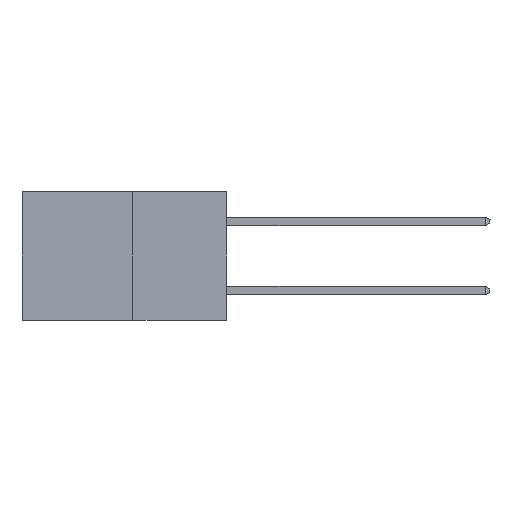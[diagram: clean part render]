
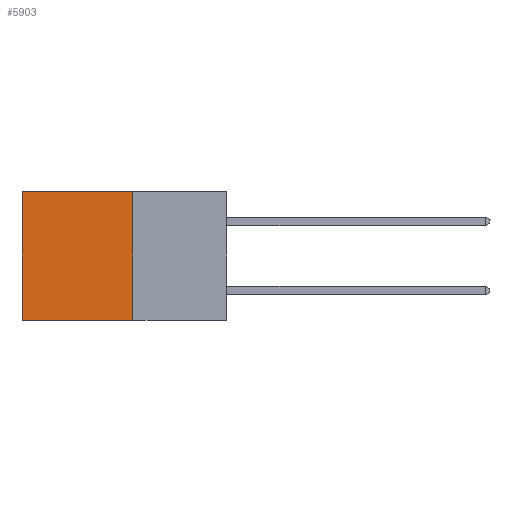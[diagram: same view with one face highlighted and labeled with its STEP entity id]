
A CAD part, left-side view. The second image highlights one B-rep face of the part: STEP entity #5903.
In plain terms, the highlighted planar face has unit normal (-1, 0, 0).
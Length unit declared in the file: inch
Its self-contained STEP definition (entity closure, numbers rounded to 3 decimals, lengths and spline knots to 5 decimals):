
#165 = EDGE_LOOP ( 'NONE', ( #9547, #2135, #2432, #10112 ) ) ;
#430 = DIRECTION ( 'NONE',  ( 0., 1., 0. ) ) ;
#759 = LINE ( 'NONE', #11367, #5685 ) ;
#804 = CARTESIAN_POINT ( 'NONE',  ( 0.277, 0.59, 0. ) ) ;
#1300 = VERTEX_POINT ( 'NONE', #804 ) ;
#1862 = CARTESIAN_POINT ( 'NONE',  ( 0.277, 0.27, -0.37 ) ) ;
#2135 = ORIENTED_EDGE ( 'NONE', *, *, #11477, .F. ) ;
#2406 = EDGE_CURVE ( 'NONE', #11969, #7955, #6826, .T. ) ;
#2407 = CARTESIAN_POINT ( 'NONE',  ( 0.277, 0.27, 0. ) ) ;
#2432 = ORIENTED_EDGE ( 'NONE', *, *, #2406, .F. ) ;
#3671 = DIRECTION ( 'NONE',  ( 0., 0., -1. ) ) ;
#3818 = DIRECTION ( 'NONE',  ( 1., 0., 0. ) ) ;
#5685 = VECTOR ( 'NONE', #10441, 39.37008 ) ;
#5777 = CARTESIAN_POINT ( 'NONE',  ( 0.277, 0.27, -0.37 ) ) ;
#5903 = ADVANCED_FACE ( 'NONE', ( #11142 ), #9595, .F. ) ;
#5915 = AXIS2_PLACEMENT_3D ( 'NONE', #1862, #3818, #10507 ) ;
#6053 = EDGE_CURVE ( 'NONE', #1300, #9940, #9114, .T. ) ;
#6290 = VECTOR ( 'NONE', #430, 39.37008 ) ;
#6358 = CARTESIAN_POINT ( 'NONE',  ( 0.277, 0.27, 0. ) ) ;
#6826 = LINE ( 'NONE', #7202, #11799 ) ;
#6969 = CARTESIAN_POINT ( 'NONE',  ( 0.277, 0.59, -0.37 ) ) ;
#7202 = CARTESIAN_POINT ( 'NONE',  ( 0.277, 0.27, -0.37 ) ) ;
#7955 = VERTEX_POINT ( 'NONE', #5777 ) ;
#8528 = LINE ( 'NONE', #6358, #6290 ) ;
#8804 = VECTOR ( 'NONE', #11646, 39.37008 ) ;
#9114 = LINE ( 'NONE', #6969, #8804 ) ;
#9547 = ORIENTED_EDGE ( 'NONE', *, *, #6053, .T. ) ;
#9595 = PLANE ( 'NONE',  #5915 ) ;
#9940 = VERTEX_POINT ( 'NONE', #10035 ) ;
#10035 = CARTESIAN_POINT ( 'NONE',  ( 0.277, 0.59, -0.37 ) ) ;
#10112 = ORIENTED_EDGE ( 'NONE', *, *, #12009, .T. ) ;
#10441 = DIRECTION ( 'NONE',  ( 0., 1., 0. ) ) ;
#10507 = DIRECTION ( 'NONE',  ( 0., 0., -1. ) ) ;
#11142 = FACE_OUTER_BOUND ( 'NONE', #165, .T. ) ;
#11367 = CARTESIAN_POINT ( 'NONE',  ( 0.277, 0.27, -0.37 ) ) ;
#11477 = EDGE_CURVE ( 'NONE', #7955, #9940, #759, .T. ) ;
#11646 = DIRECTION ( 'NONE',  ( 0., 0., -1. ) ) ;
#11799 = VECTOR ( 'NONE', #3671, 39.37008 ) ;
#11969 = VERTEX_POINT ( 'NONE', #2407 ) ;
#12009 = EDGE_CURVE ( 'NONE', #11969, #1300, #8528, .T. ) ;
